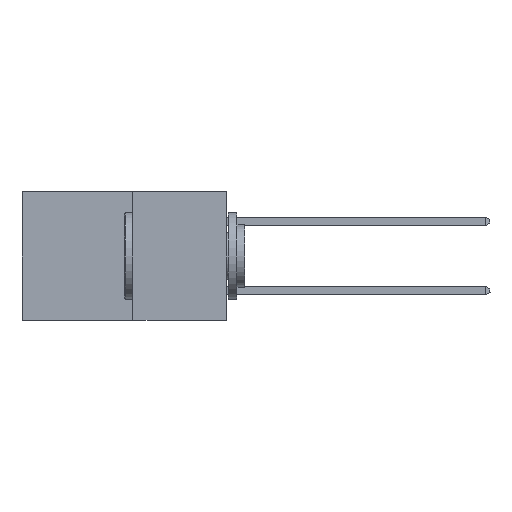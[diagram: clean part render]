
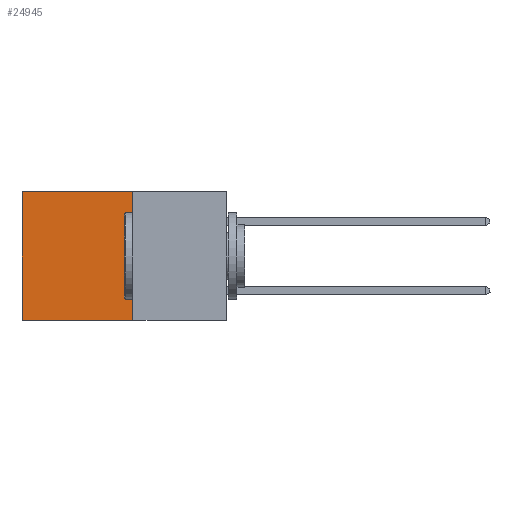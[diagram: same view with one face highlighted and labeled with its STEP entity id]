
A CAD part, left-side view. The second image highlights one B-rep face of the part: STEP entity #24945.
In plain terms, the highlighted planar face has unit normal (-1, 0, 0).
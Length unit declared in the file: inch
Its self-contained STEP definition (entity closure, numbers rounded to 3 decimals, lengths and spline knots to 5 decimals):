
#718 = EDGE_CURVE ( 'NONE', #26774, #26104, #4384, .T. ) ;
#748 = CARTESIAN_POINT ( 'NONE',  ( 0.277, 0.59, -0.37 ) ) ;
#1028 = ORIENTED_EDGE ( 'NONE', *, *, #28871, .F. ) ;
#1513 = CARTESIAN_POINT ( 'NONE',  ( 0.277, 0.59, -0.37 ) ) ;
#3362 = DIRECTION ( 'NONE',  ( 0., 0., -1. ) ) ;
#3609 = VECTOR ( 'NONE', #21080, 39.37008 ) ;
#3908 = CARTESIAN_POINT ( 'NONE',  ( 0.277, 0.27, -0.37 ) ) ;
#4214 = VERTEX_POINT ( 'NONE', #20737 ) ;
#4384 = LINE ( 'NONE', #27024, #16493 ) ;
#4722 = EDGE_CURVE ( 'NONE', #4214, #17443, #16484, .T. ) ;
#4980 = VECTOR ( 'NONE', #11264, 39.37008 ) ;
#5253 = CARTESIAN_POINT ( 'NONE',  ( 0.277, 0.27, -0.37 ) ) ;
#5734 = LINE ( 'NONE', #1513, #4980 ) ;
#6342 = DIRECTION ( 'NONE',  ( 0., 0., -1. ) ) ;
#8683 = PLANE ( 'NONE',  #12893 ) ;
#10786 = CARTESIAN_POINT ( 'NONE',  ( 0.277, 0.27, 0. ) ) ;
#11264 = DIRECTION ( 'NONE',  ( 0., 0., -1. ) ) ;
#11911 = VECTOR ( 'NONE', #3362, 39.37008 ) ;
#12893 = AXIS2_PLACEMENT_3D ( 'NONE', #3908, #20764, #6342 ) ;
#13644 = EDGE_LOOP ( 'NONE', ( #26714, #22365, #1028, #27865 ) ) ;
#16484 = LINE ( 'NONE', #5253, #3609 ) ;
#16493 = VECTOR ( 'NONE', #23676, 39.37008 ) ;
#17443 = VERTEX_POINT ( 'NONE', #748 ) ;
#20219 = CARTESIAN_POINT ( 'NONE',  ( 0.277, 0.27, -0.37 ) ) ;
#20292 = EDGE_CURVE ( 'NONE', #26104, #17443, #5734, .T. ) ;
#20737 = CARTESIAN_POINT ( 'NONE',  ( 0.277, 0.27, -0.37 ) ) ;
#20764 = DIRECTION ( 'NONE',  ( 1., 0., 0. ) ) ;
#21080 = DIRECTION ( 'NONE',  ( 0., 1., 0. ) ) ;
#22365 = ORIENTED_EDGE ( 'NONE', *, *, #4722, .F. ) ;
#23676 = DIRECTION ( 'NONE',  ( 0., 1., 0. ) ) ;
#24945 = ADVANCED_FACE ( 'NONE', ( #27842 ), #8683, .F. ) ;
#25080 = CARTESIAN_POINT ( 'NONE',  ( 0.277, 0.59, 0. ) ) ;
#26104 = VERTEX_POINT ( 'NONE', #25080 ) ;
#26714 = ORIENTED_EDGE ( 'NONE', *, *, #20292, .T. ) ;
#26774 = VERTEX_POINT ( 'NONE', #10786 ) ;
#27024 = CARTESIAN_POINT ( 'NONE',  ( 0.277, 0.27, 0. ) ) ;
#27842 = FACE_OUTER_BOUND ( 'NONE', #13644, .T. ) ;
#27865 = ORIENTED_EDGE ( 'NONE', *, *, #718, .T. ) ;
#28871 = EDGE_CURVE ( 'NONE', #26774, #4214, #30249, .T. ) ;
#30249 = LINE ( 'NONE', #20219, #11911 ) ;
